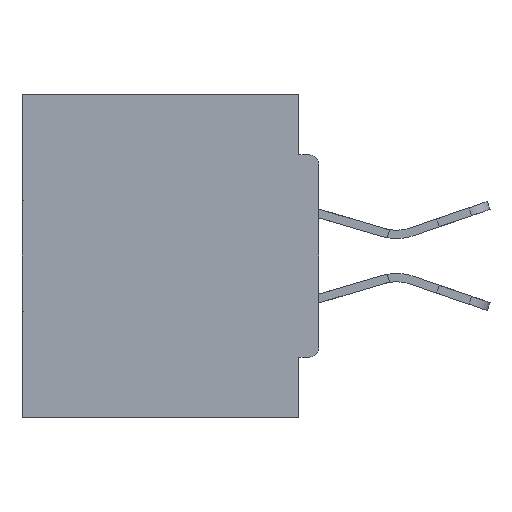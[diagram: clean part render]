
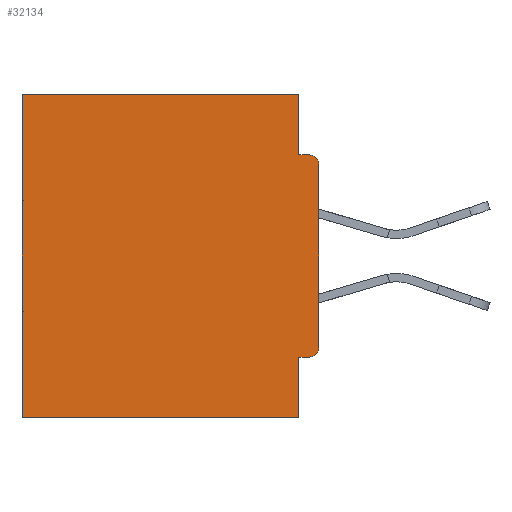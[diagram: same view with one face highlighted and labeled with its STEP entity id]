
A CAD part, left-side view. The second image highlights one B-rep face of the part: STEP entity #32134.
In plain terms, the highlighted planar face has unit normal (-1, 0, 0).
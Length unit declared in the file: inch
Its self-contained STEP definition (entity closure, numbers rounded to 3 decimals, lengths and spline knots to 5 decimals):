
#1044 = VECTOR ( 'NONE', #29570, 39.37008 ) ;
#1620 = CARTESIAN_POINT ( 'NONE',  ( 0.298, 0., -0.3915 ) ) ;
#1815 = CARTESIAN_POINT ( 'NONE',  ( 0.298, 0.031, -0.5 ) ) ;
#2304 = EDGE_LOOP ( 'NONE', ( #7287, #22816, #16221, #2318, #23064, #31700, #5483, #13426, #31461, #26263 ) ) ;
#2318 = ORIENTED_EDGE ( 'NONE', *, *, #19542, .T. ) ;
#3198 = VERTEX_POINT ( 'NONE', #42222 ) ;
#3699 = EDGE_CURVE ( 'NONE', #34557, #3708, #21762, .T. ) ;
#3708 = VERTEX_POINT ( 'NONE', #36147 ) ;
#3839 = EDGE_CURVE ( 'NONE', #35912, #40164, #35733, .T. ) ;
#5273 = DIRECTION ( 'NONE',  ( 0., 0., -1. ) ) ;
#5483 = ORIENTED_EDGE ( 'NONE', *, *, #14303, .F. ) ;
#5583 = DIRECTION ( 'NONE',  ( 0., 0., -1. ) ) ;
#5621 = CIRCLE ( 'NONE', #18945, 0.015 ) ;
#6385 = LINE ( 'NONE', #31652, #29744 ) ;
#7267 = CARTESIAN_POINT ( 'NONE',  ( 0.298, 0., 0. ) ) ;
#7287 = ORIENTED_EDGE ( 'NONE', *, *, #34356, .T. ) ;
#7744 = CARTESIAN_POINT ( 'NONE',  ( 0.298, 0.46, 0. ) ) ;
#8423 = LINE ( 'NONE', #32451, #37049 ) ;
#8862 = DIRECTION ( 'NONE',  ( 0., 0., -1. ) ) ;
#9047 = DIRECTION ( 'NONE',  ( 0., 0., -1. ) ) ;
#9195 = CARTESIAN_POINT ( 'NONE',  ( 0.298, 0.015, -0.1085 ) ) ;
#9577 = EDGE_CURVE ( 'NONE', #36039, #32366, #36630, .T. ) ;
#11060 = CARTESIAN_POINT ( 'NONE',  ( 0.298, 0., -0.4065 ) ) ;
#11203 = VECTOR ( 'NONE', #35135, 39.37008 ) ;
#11634 = CARTESIAN_POINT ( 'NONE',  ( 0.298, 0., 0. ) ) ;
#12583 = EDGE_CURVE ( 'NONE', #36355, #3708, #21800, .T. ) ;
#12912 = VECTOR ( 'NONE', #19902, 39.37008 ) ;
#13146 = CARTESIAN_POINT ( 'NONE',  ( 0.298, 0., -0.5 ) ) ;
#13426 = ORIENTED_EDGE ( 'NONE', *, *, #22521, .F. ) ;
#14303 = EDGE_CURVE ( 'NONE', #35596, #36355, #8423, .T. ) ;
#14569 = EDGE_CURVE ( 'NONE', #3198, #36039, #18845, .T. ) ;
#15843 = DIRECTION ( 'NONE',  ( -1., 0., 0. ) ) ;
#16221 = ORIENTED_EDGE ( 'NONE', *, *, #14569, .F. ) ;
#16397 = CARTESIAN_POINT ( 'NONE',  ( 0.298, 0.46, 0. ) ) ;
#17000 = LINE ( 'NONE', #11060, #23765 ) ;
#18433 = PLANE ( 'NONE',  #35403 ) ;
#18845 = LINE ( 'NONE', #1815, #42186 ) ;
#18937 = DIRECTION ( 'NONE',  ( 0., 0., -1. ) ) ;
#18945 = AXIS2_PLACEMENT_3D ( 'NONE', #9195, #19231, #9047 ) ;
#19222 = CIRCLE ( 'NONE', #21778, 0.015 ) ;
#19231 = DIRECTION ( 'NONE',  ( -1., 0., 0. ) ) ;
#19542 = EDGE_CURVE ( 'NONE', #3198, #34557, #6385, .T. ) ;
#19902 = DIRECTION ( 'NONE',  ( 0., 0., -1. ) ) ;
#20559 = EDGE_CURVE ( 'NONE', #26257, #40164, #19222, .T. ) ;
#21762 = LINE ( 'NONE', #16397, #12912 ) ;
#21778 = AXIS2_PLACEMENT_3D ( 'NONE', #22239, #15843, #8862 ) ;
#21800 = LINE ( 'NONE', #13146, #1044 ) ;
#22239 = CARTESIAN_POINT ( 'NONE',  ( 0.298, 0.015, -0.3915 ) ) ;
#22488 = CARTESIAN_POINT ( 'NONE',  ( 0.298, 0.031, -0.0935 ) ) ;
#22521 = EDGE_CURVE ( 'NONE', #26257, #35596, #17000, .T. ) ;
#22816 = ORIENTED_EDGE ( 'NONE', *, *, #9577, .F. ) ;
#23064 = ORIENTED_EDGE ( 'NONE', *, *, #3699, .T. ) ;
#23765 = VECTOR ( 'NONE', #33964, 39.37008 ) ;
#24570 = CARTESIAN_POINT ( 'NONE',  ( 0.298, 0., -0.1085 ) ) ;
#25176 = CARTESIAN_POINT ( 'NONE',  ( 0.298, 0., -0.0935 ) ) ;
#26257 = VERTEX_POINT ( 'NONE', #41102 ) ;
#26263 = ORIENTED_EDGE ( 'NONE', *, *, #3839, .F. ) ;
#27685 = CARTESIAN_POINT ( 'NONE',  ( 0.298, 0.031, -0.4065 ) ) ;
#28621 = DIRECTION ( 'NONE',  ( 1., 0., 0. ) ) ;
#29570 = DIRECTION ( 'NONE',  ( 0., 1., 0. ) ) ;
#29744 = VECTOR ( 'NONE', #34852, 39.37008 ) ;
#30507 = DIRECTION ( 'NONE',  ( 0., 0., -1. ) ) ;
#31156 = FACE_OUTER_BOUND ( 'NONE', #2304, .T. ) ;
#31461 = ORIENTED_EDGE ( 'NONE', *, *, #20559, .T. ) ;
#31652 = CARTESIAN_POINT ( 'NONE',  ( 0.298, 0., 0. ) ) ;
#31700 = ORIENTED_EDGE ( 'NONE', *, *, #12583, .F. ) ;
#31867 = CARTESIAN_POINT ( 'NONE',  ( 0.298, 0.031, -0.5 ) ) ;
#32134 = ADVANCED_FACE ( 'NONE', ( #31156 ), #18433, .F. ) ;
#32366 = VERTEX_POINT ( 'NONE', #36817 ) ;
#32451 = CARTESIAN_POINT ( 'NONE',  ( 0.298, 0.031, -0.5 ) ) ;
#33964 = DIRECTION ( 'NONE',  ( 0., 1., 0. ) ) ;
#34356 = EDGE_CURVE ( 'NONE', #35912, #32366, #5621, .T. ) ;
#34557 = VERTEX_POINT ( 'NONE', #7744 ) ;
#34852 = DIRECTION ( 'NONE',  ( 0., 1., 0. ) ) ;
#35135 = DIRECTION ( 'NONE',  ( 0., -1., 0. ) ) ;
#35403 = AXIS2_PLACEMENT_3D ( 'NONE', #11634, #28621, #5273 ) ;
#35596 = VERTEX_POINT ( 'NONE', #27685 ) ;
#35733 = LINE ( 'NONE', #7267, #40909 ) ;
#35912 = VERTEX_POINT ( 'NONE', #24570 ) ;
#36039 = VERTEX_POINT ( 'NONE', #22488 ) ;
#36147 = CARTESIAN_POINT ( 'NONE',  ( 0.298, 0.46, -0.5 ) ) ;
#36355 = VERTEX_POINT ( 'NONE', #31867 ) ;
#36630 = LINE ( 'NONE', #25176, #11203 ) ;
#36817 = CARTESIAN_POINT ( 'NONE',  ( 0.298, 0.015, -0.0935 ) ) ;
#37049 = VECTOR ( 'NONE', #18937, 39.37008 ) ;
#40164 = VERTEX_POINT ( 'NONE', #1620 ) ;
#40909 = VECTOR ( 'NONE', #30507, 39.37008 ) ;
#41102 = CARTESIAN_POINT ( 'NONE',  ( 0.298, 0.015, -0.4065 ) ) ;
#42186 = VECTOR ( 'NONE', #5583, 39.37008 ) ;
#42222 = CARTESIAN_POINT ( 'NONE',  ( 0.298, 0.031, 0. ) ) ;
